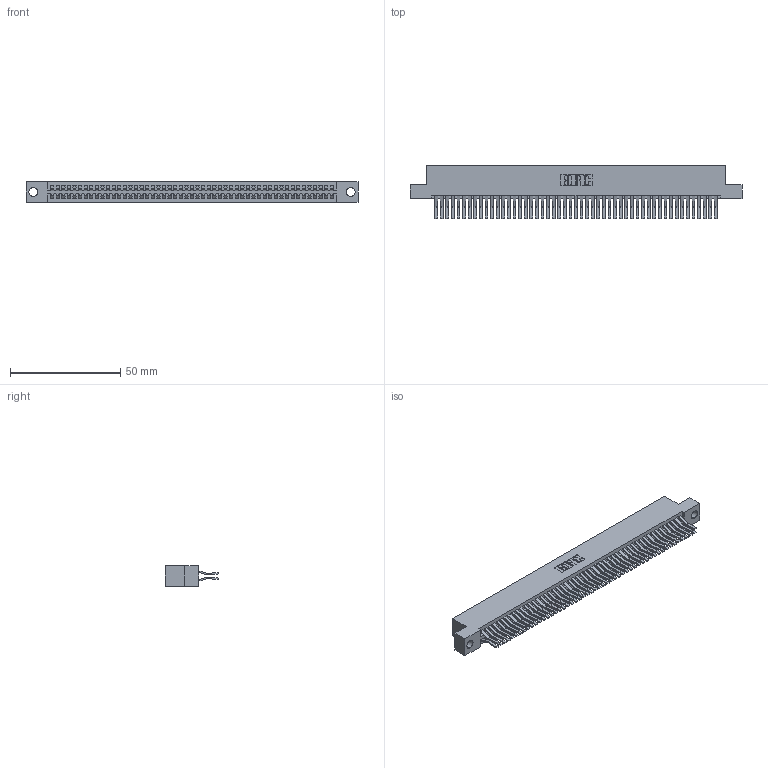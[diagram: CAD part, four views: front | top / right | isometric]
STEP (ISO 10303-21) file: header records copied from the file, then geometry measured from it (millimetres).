
FILE_DESCRIPTION (( 'STEP AP203' ), '1' );
FILE_NAME ('395-102-560-204.STEP', '2021-06-17T15:49:58', ( '' ), ( '' ), 'SwSTEP 2.0', 'SolidWorks 2020', '' );
FILE_SCHEMA (( 'CONFIG_CONTROL_DESIGN' ));
Length unit declared in the file: inch
Products named in the file (3): 345 Part_Flush Mounting Lugs - 0.156 Dia-TI; 395-102-560-204; 345-292-001_560 Tail
Assembly tree (103 placements, depth 2):
  395-102-560-204
    345 Part_Flush Mounting Lugs - 0.156 Dia-TI
    345-292-001_560 Tail  x102
Bounding box: 150.75 x 24.45 x 9.4 mm (x, y, z)
Volume: 15290.1 mm3; surface area: 24346.7 mm2
Topology: 103 solids, 103 shells, 5444 faces, 16187 edges, 10654 vertices
Faces by surface type: plane 3460, cylinder 1984
Entity records: 39311 total; most frequent: CARTESIAN_POINT 6586, ORIENTED_EDGE 6518, DIRECTION 5799, EDGE_CURVE 3259, LINE 2919, VECTOR 2919, VERTEX_POINT 2170, AXIS2_PLACEMENT_3D 1440
